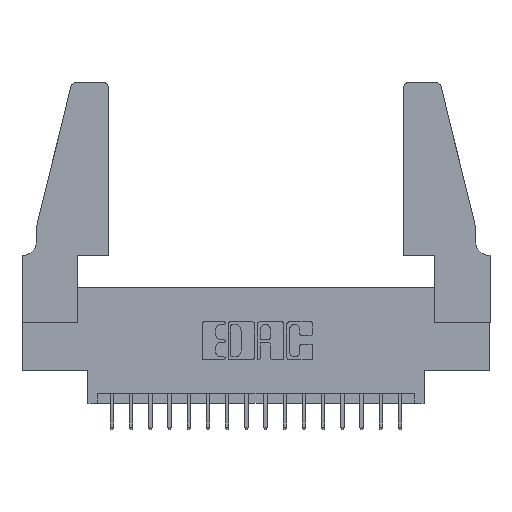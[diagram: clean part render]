
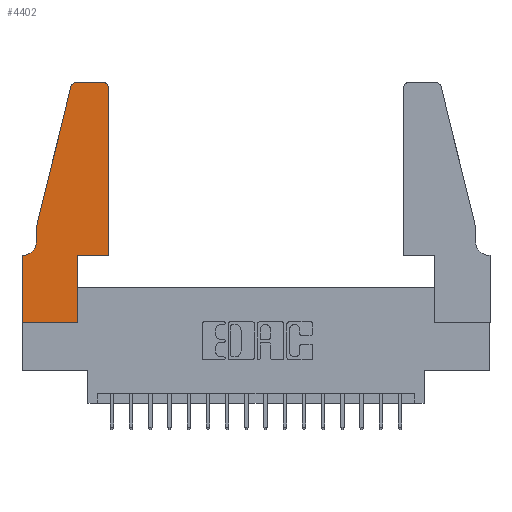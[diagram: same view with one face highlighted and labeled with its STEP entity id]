
A CAD part, top view. The second image highlights one B-rep face of the part: STEP entity #4402.
In plain terms, the highlighted planar face has unit normal (0, 0, 1).
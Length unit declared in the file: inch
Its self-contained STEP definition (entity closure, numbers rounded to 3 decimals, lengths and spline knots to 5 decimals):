
#23 = ORIENTED_EDGE ( 'NONE', *, *, #17747, .T. ) ;
#46 = CARTESIAN_POINT ( 'NONE',  ( 0.2865, 0., 0.37 ) ) ;
#126 = DIRECTION ( 'NONE',  ( 0., 0., 1. ) ) ;
#133 = ORIENTED_EDGE ( 'NONE', *, *, #9781, .T. ) ;
#302 = ORIENTED_EDGE ( 'NONE', *, *, #2659, .T. ) ;
#433 = LINE ( 'NONE', #10520, #7185 ) ;
#491 = AXIS2_PLACEMENT_3D ( 'NONE', #15493, #7930, #13742 ) ;
#514 = CARTESIAN_POINT ( 'NONE',  ( 0.0055, 0.35, 0.37 ) ) ;
#876 = DIRECTION ( 'NONE',  ( -1., 0., 0. ) ) ;
#1083 = VECTOR ( 'NONE', #12372, 39.37008 ) ;
#1312 = CARTESIAN_POINT ( 'NONE',  ( 0.2605, 1.25, 0.37 ) ) ;
#1602 = ORIENTED_EDGE ( 'NONE', *, *, #6029, .T. ) ;
#1664 = VECTOR ( 'NONE', #9432, 39.37008 ) ;
#1931 = VECTOR ( 'NONE', #4794, 39.37008 ) ;
#1979 = CARTESIAN_POINT ( 'NONE',  ( 0.4505, 0.35, 0.37 ) ) ;
#2074 = VECTOR ( 'NONE', #3951, 39.37008 ) ;
#2357 = CARTESIAN_POINT ( 'NONE',  ( 0.0755, 0.35, 0.37 ) ) ;
#2367 = LINE ( 'NONE', #13785, #1083 ) ;
#2544 = ORIENTED_EDGE ( 'NONE', *, *, #5160, .T. ) ;
#2659 = EDGE_CURVE ( 'NONE', #11106, #7913, #10619, .T. ) ;
#2757 = ORIENTED_EDGE ( 'NONE', *, *, #11019, .T. ) ;
#3744 = CARTESIAN_POINT ( 'NONE',  ( 0.0755, 0.42, 0.37 ) ) ;
#3861 = LINE ( 'NONE', #1312, #2074 ) ;
#3951 = DIRECTION ( 'NONE',  ( -1., 0., 0. ) ) ;
#3952 = EDGE_CURVE ( 'NONE', #16891, #17305, #10086, .T. ) ;
#4106 = CARTESIAN_POINT ( 'NONE',  ( 0.284, 1.22, 0.37 ) ) ;
#4402 = ADVANCED_FACE ( 'NONE', ( #9496 ), #10904, .T. ) ;
#4542 = ORIENTED_EDGE ( 'NONE', *, *, #12067, .T. ) ;
#4626 = DIRECTION ( 'NONE',  ( 1., 0., 0. ) ) ;
#4644 = LINE ( 'NONE', #17784, #9557 ) ;
#4794 = DIRECTION ( 'NONE',  ( 0., 1., 0. ) ) ;
#5160 = EDGE_CURVE ( 'NONE', #13604, #14786, #14504, .T. ) ;
#5815 = DIRECTION ( 'NONE',  ( 1., 0., 0. ) ) ;
#6029 = EDGE_CURVE ( 'NONE', #17305, #10350, #433, .T. ) ;
#6143 = EDGE_CURVE ( 'NONE', #14158, #12941, #4644, .T. ) ;
#6375 = ORIENTED_EDGE ( 'NONE', *, *, #12277, .T. ) ;
#6638 = LINE ( 'NONE', #13654, #1664 ) ;
#6774 = EDGE_CURVE ( 'NONE', #7913, #14158, #15055, .T. ) ;
#6868 = CARTESIAN_POINT ( 'NONE',  ( 0.4505, 1.22, 0.37 ) ) ;
#7098 = AXIS2_PLACEMENT_3D ( 'NONE', #15287, #8377, #13898 ) ;
#7185 = VECTOR ( 'NONE', #7521, 39.37008 ) ;
#7212 = CARTESIAN_POINT ( 'NONE',  ( 0.4205, 1.22, 0.37 ) ) ;
#7409 = VECTOR ( 'NONE', #14685, 39.37008 ) ;
#7507 = LINE ( 'NONE', #11805, #9252 ) ;
#7521 = DIRECTION ( 'NONE',  ( -0.239, -0.971, 0. ) ) ;
#7913 = VERTEX_POINT ( 'NONE', #514 ) ;
#7930 = DIRECTION ( 'NONE',  ( 0., 0., -1. ) ) ;
#8117 = CARTESIAN_POINT ( 'NONE',  ( 0., 0.35, 0.37 ) ) ;
#8205 = AXIS2_PLACEMENT_3D ( 'NONE', #7212, #126, #5815 ) ;
#8377 = DIRECTION ( 'NONE',  ( 0., 0., 1. ) ) ;
#9252 = VECTOR ( 'NONE', #4626, 39.37008 ) ;
#9269 = VERTEX_POINT ( 'NONE', #13239 ) ;
#9432 = DIRECTION ( 'NONE',  ( 0., -1., 0. ) ) ;
#9496 = FACE_OUTER_BOUND ( 'NONE', #13485, .T. ) ;
#9557 = VECTOR ( 'NONE', #17503, 39.37008 ) ;
#9781 = EDGE_CURVE ( 'NONE', #12040, #16505, #11786, .T. ) ;
#9980 = ORIENTED_EDGE ( 'NONE', *, *, #6774, .T. ) ;
#10086 = CIRCLE ( 'NONE', #13355, 0.03 ) ;
#10350 = VERTEX_POINT ( 'NONE', #14105 ) ;
#10520 = CARTESIAN_POINT ( 'NONE',  ( 0.0755, 0.5, 0.37 ) ) ;
#10619 = CIRCLE ( 'NONE', #491, 0.07 ) ;
#10904 = PLANE ( 'NONE',  #7098 ) ;
#11019 = EDGE_CURVE ( 'NONE', #12941, #12040, #2367, .T. ) ;
#11106 = VERTEX_POINT ( 'NONE', #3744 ) ;
#11116 = DIRECTION ( 'NONE',  ( 0., 0., 1. ) ) ;
#11461 = CARTESIAN_POINT ( 'NONE',  ( 0., 0., 0.37 ) ) ;
#11786 = LINE ( 'NONE', #14684, #1931 ) ;
#11805 = CARTESIAN_POINT ( 'NONE',  ( 0.4505, 0.35, 0.37 ) ) ;
#11872 = ORIENTED_EDGE ( 'NONE', *, *, #3952, .T. ) ;
#12040 = VERTEX_POINT ( 'NONE', #46 ) ;
#12067 = EDGE_CURVE ( 'NONE', #14786, #9269, #16237, .T. ) ;
#12277 = EDGE_CURVE ( 'NONE', #10350, #11106, #6638, .T. ) ;
#12372 = DIRECTION ( 'NONE',  ( 1., 0., 0. ) ) ;
#12941 = VERTEX_POINT ( 'NONE', #11461 ) ;
#13239 = CARTESIAN_POINT ( 'NONE',  ( 0.4205, 1.25, 0.37 ) ) ;
#13355 = AXIS2_PLACEMENT_3D ( 'NONE', #4106, #11116, #16790 ) ;
#13485 = EDGE_LOOP ( 'NONE', ( #17082, #11872, #1602, #6375, #302, #9980, #14905, #2757, #133, #23, #2544, #4542 ) ) ;
#13604 = VERTEX_POINT ( 'NONE', #15044 ) ;
#13654 = CARTESIAN_POINT ( 'NONE',  ( 0.0755, 0.5, 0.37 ) ) ;
#13742 = DIRECTION ( 'NONE',  ( -1., 0., 0. ) ) ;
#13785 = CARTESIAN_POINT ( 'NONE',  ( 0., 0., 0.37 ) ) ;
#13898 = DIRECTION ( 'NONE',  ( 1., 0., 0. ) ) ;
#14014 = VECTOR ( 'NONE', #876, 39.37008 ) ;
#14105 = CARTESIAN_POINT ( 'NONE',  ( 0.0755, 0.5, 0.37 ) ) ;
#14158 = VERTEX_POINT ( 'NONE', #8117 ) ;
#14471 = CARTESIAN_POINT ( 'NONE',  ( 0.25487, 1.22718, 0.37 ) ) ;
#14504 = LINE ( 'NONE', #1979, #7409 ) ;
#14684 = CARTESIAN_POINT ( 'NONE',  ( 0.2865, 0.35, 0.37 ) ) ;
#14685 = DIRECTION ( 'NONE',  ( 0., 1., 0. ) ) ;
#14786 = VERTEX_POINT ( 'NONE', #6868 ) ;
#14905 = ORIENTED_EDGE ( 'NONE', *, *, #6143, .T. ) ;
#15044 = CARTESIAN_POINT ( 'NONE',  ( 0.4505, 0.35, 0.37 ) ) ;
#15055 = LINE ( 'NONE', #2357, #14014 ) ;
#15166 = CARTESIAN_POINT ( 'NONE',  ( 0.2865, 0.35, 0.37 ) ) ;
#15287 = CARTESIAN_POINT ( 'NONE',  ( 0., 0.35, 0.37 ) ) ;
#15493 = CARTESIAN_POINT ( 'NONE',  ( 0.0055, 0.42, 0.37 ) ) ;
#16237 = CIRCLE ( 'NONE', #8205, 0.03 ) ;
#16505 = VERTEX_POINT ( 'NONE', #15166 ) ;
#16790 = DIRECTION ( 'NONE',  ( 1., 0., 0. ) ) ;
#16891 = VERTEX_POINT ( 'NONE', #17372 ) ;
#17082 = ORIENTED_EDGE ( 'NONE', *, *, #18429, .T. ) ;
#17305 = VERTEX_POINT ( 'NONE', #14471 ) ;
#17372 = CARTESIAN_POINT ( 'NONE',  ( 0.284, 1.25, 0.37 ) ) ;
#17503 = DIRECTION ( 'NONE',  ( 0., -1., 0. ) ) ;
#17747 = EDGE_CURVE ( 'NONE', #16505, #13604, #7507, .T. ) ;
#17784 = CARTESIAN_POINT ( 'NONE',  ( 0., 0., 0.37 ) ) ;
#18429 = EDGE_CURVE ( 'NONE', #9269, #16891, #3861, .T. ) ;
